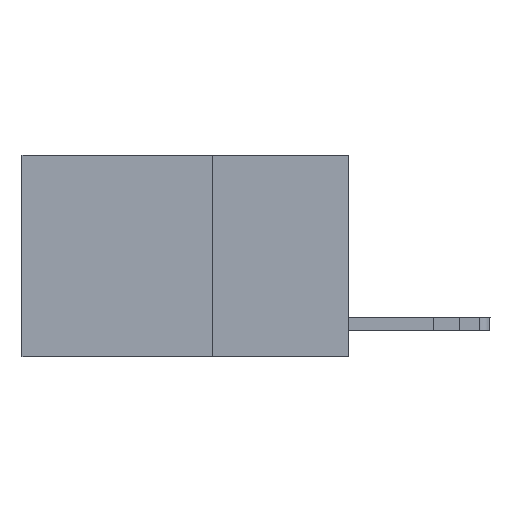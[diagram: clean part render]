
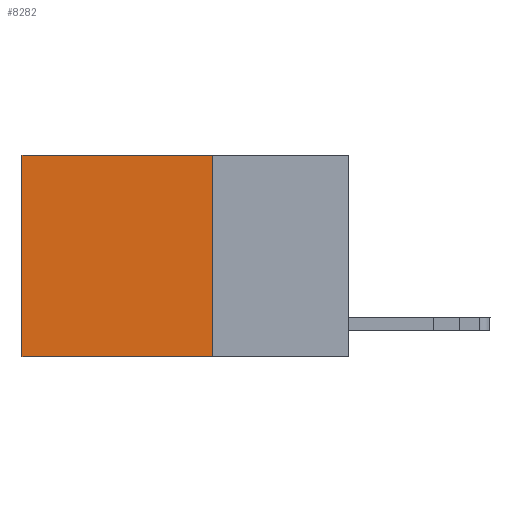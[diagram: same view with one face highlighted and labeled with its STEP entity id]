
A CAD part, left-side view. The second image highlights one B-rep face of the part: STEP entity #8282.
In plain terms, the highlighted planar face has unit normal (-1, 0, 0).
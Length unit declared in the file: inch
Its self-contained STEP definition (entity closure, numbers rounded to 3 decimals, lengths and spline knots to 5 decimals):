
#1317 = VERTEX_POINT ( 'NONE', #14596 ) ;
#1423 = DIRECTION ( 'NONE',  ( 0., 1., 0. ) ) ;
#3292 = DIRECTION ( 'NONE',  ( 0., 0., -1. ) ) ;
#3715 = AXIS2_PLACEMENT_3D ( 'NONE', #16153, #19517, #12875 ) ;
#3875 = EDGE_CURVE ( 'NONE', #15819, #8160, #4936, .T. ) ;
#4529 = EDGE_CURVE ( 'NONE', #6580, #8160, #4675, .T. ) ;
#4675 = LINE ( 'NONE', #15375, #6633 ) ;
#4766 = CARTESIAN_POINT ( 'NONE',  ( 0.2625, 0.6, -0.37 ) ) ;
#4936 = LINE ( 'NONE', #11109, #9528 ) ;
#6580 = VERTEX_POINT ( 'NONE', #8807 ) ;
#6633 = VECTOR ( 'NONE', #1423, 39.37008 ) ;
#8160 = VERTEX_POINT ( 'NONE', #4766 ) ;
#8282 = ADVANCED_FACE ( 'NONE', ( #16468 ), #13281, .F. ) ;
#8807 = CARTESIAN_POINT ( 'NONE',  ( 0.2625, 0.25, -0.37 ) ) ;
#9528 = VECTOR ( 'NONE', #3292, 39.37008 ) ;
#9631 = VECTOR ( 'NONE', #15532, 39.37008 ) ;
#9918 = EDGE_CURVE ( 'NONE', #1317, #6580, #10838, .T. ) ;
#9975 = EDGE_CURVE ( 'NONE', #1317, #15819, #17277, .T. ) ;
#10838 = LINE ( 'NONE', #17457, #14175 ) ;
#11109 = CARTESIAN_POINT ( 'NONE',  ( 0.2625, 0.6, 0. ) ) ;
#12448 = ORIENTED_EDGE ( 'NONE', *, *, #9918, .F. ) ;
#12678 = EDGE_LOOP ( 'NONE', ( #17027, #16014, #12448, #19742 ) ) ;
#12875 = DIRECTION ( 'NONE',  ( 0., 0., -1. ) ) ;
#13281 = PLANE ( 'NONE',  #3715 ) ;
#14147 = CARTESIAN_POINT ( 'NONE',  ( 0.2625, 0.6, 0. ) ) ;
#14175 = VECTOR ( 'NONE', #19090, 39.37008 ) ;
#14596 = CARTESIAN_POINT ( 'NONE',  ( 0.2625, 0.25, 0. ) ) ;
#15375 = CARTESIAN_POINT ( 'NONE',  ( 0.2625, 0.25, -0.37 ) ) ;
#15532 = DIRECTION ( 'NONE',  ( 0., 1., 0. ) ) ;
#15819 = VERTEX_POINT ( 'NONE', #14147 ) ;
#16014 = ORIENTED_EDGE ( 'NONE', *, *, #4529, .F. ) ;
#16153 = CARTESIAN_POINT ( 'NONE',  ( 0.2625, 0.25, 0. ) ) ;
#16468 = FACE_OUTER_BOUND ( 'NONE', #12678, .T. ) ;
#17027 = ORIENTED_EDGE ( 'NONE', *, *, #3875, .T. ) ;
#17277 = LINE ( 'NONE', #18801, #9631 ) ;
#17457 = CARTESIAN_POINT ( 'NONE',  ( 0.2625, 0.25, 0. ) ) ;
#18801 = CARTESIAN_POINT ( 'NONE',  ( 0.2625, 0.25, 0. ) ) ;
#19090 = DIRECTION ( 'NONE',  ( 0., 0., -1. ) ) ;
#19517 = DIRECTION ( 'NONE',  ( 1., 0., 0. ) ) ;
#19742 = ORIENTED_EDGE ( 'NONE', *, *, #9975, .T. ) ;
